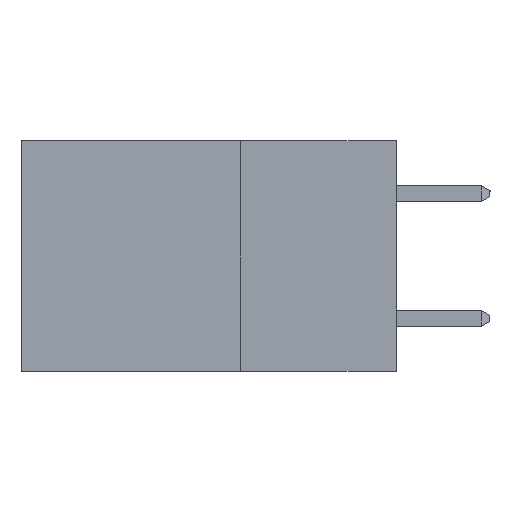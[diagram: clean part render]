
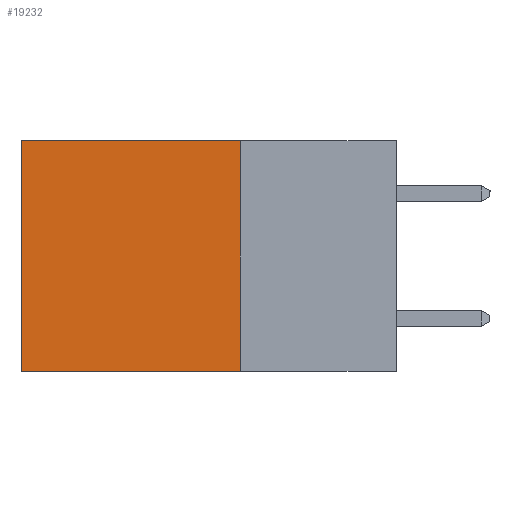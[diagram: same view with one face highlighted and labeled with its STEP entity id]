
A CAD part, left-side view. The second image highlights one B-rep face of the part: STEP entity #19232.
In plain terms, the highlighted planar face has unit normal (-1, 0, 0).
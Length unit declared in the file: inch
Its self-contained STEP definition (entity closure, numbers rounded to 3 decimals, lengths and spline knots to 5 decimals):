
#616 = DIRECTION ( 'NONE',  ( 0., 1., 0. ) ) ;
#619 = CARTESIAN_POINT ( 'NONE',  ( 0.2615, 0.6, -0.37 ) ) ;
#862 = CARTESIAN_POINT ( 'NONE',  ( 0.2615, 0.25, 0. ) ) ;
#2485 = LINE ( 'NONE', #9546, #17303 ) ;
#2543 = CARTESIAN_POINT ( 'NONE',  ( 0.2615, 0.25, 0. ) ) ;
#2738 = CARTESIAN_POINT ( 'NONE',  ( 0.2615, 0.6, 0. ) ) ;
#3165 = LINE ( 'NONE', #12477, #15837 ) ;
#3560 = VERTEX_POINT ( 'NONE', #15612 ) ;
#4086 = DIRECTION ( 'NONE',  ( 0., 1., 0. ) ) ;
#4348 = ORIENTED_EDGE ( 'NONE', *, *, #12219, .F. ) ;
#5095 = PLANE ( 'NONE',  #7395 ) ;
#6583 = VERTEX_POINT ( 'NONE', #2738 ) ;
#6604 = VERTEX_POINT ( 'NONE', #2543 ) ;
#6844 = DIRECTION ( 'NONE',  ( 1., 0., 0. ) ) ;
#7395 = AXIS2_PLACEMENT_3D ( 'NONE', #9579, #6844, #9480 ) ;
#7943 = EDGE_CURVE ( 'NONE', #6583, #11379, #3165, .T. ) ;
#9127 = CARTESIAN_POINT ( 'NONE',  ( 0.2615, 0.25, -0.37 ) ) ;
#9480 = DIRECTION ( 'NONE',  ( 0., 0., -1. ) ) ;
#9546 = CARTESIAN_POINT ( 'NONE',  ( 0.2615, 0.25, -0.37 ) ) ;
#9579 = CARTESIAN_POINT ( 'NONE',  ( 0.2615, 0.25, -0.37 ) ) ;
#10403 = LINE ( 'NONE', #9127, #18814 ) ;
#10695 = VECTOR ( 'NONE', #4086, 39.37008 ) ;
#11290 = ORIENTED_EDGE ( 'NONE', *, *, #14383, .T. ) ;
#11379 = VERTEX_POINT ( 'NONE', #619 ) ;
#12219 = EDGE_CURVE ( 'NONE', #6604, #3560, #10403, .T. ) ;
#12477 = CARTESIAN_POINT ( 'NONE',  ( 0.2615, 0.6, -0.37 ) ) ;
#13989 = FACE_OUTER_BOUND ( 'NONE', #14093, .T. ) ;
#14093 = EDGE_LOOP ( 'NONE', ( #17635, #14641, #4348, #11290 ) ) ;
#14383 = EDGE_CURVE ( 'NONE', #6604, #6583, #15948, .T. ) ;
#14641 = ORIENTED_EDGE ( 'NONE', *, *, #16536, .F. ) ;
#15100 = DIRECTION ( 'NONE',  ( 0., 0., -1. ) ) ;
#15226 = DIRECTION ( 'NONE',  ( 0., 0., -1. ) ) ;
#15612 = CARTESIAN_POINT ( 'NONE',  ( 0.2615, 0.25, -0.37 ) ) ;
#15837 = VECTOR ( 'NONE', #15226, 39.37008 ) ;
#15948 = LINE ( 'NONE', #862, #10695 ) ;
#16536 = EDGE_CURVE ( 'NONE', #3560, #11379, #2485, .T. ) ;
#17303 = VECTOR ( 'NONE', #616, 39.37008 ) ;
#17635 = ORIENTED_EDGE ( 'NONE', *, *, #7943, .T. ) ;
#18814 = VECTOR ( 'NONE', #15100, 39.37008 ) ;
#19232 = ADVANCED_FACE ( 'NONE', ( #13989 ), #5095, .F. ) ;
